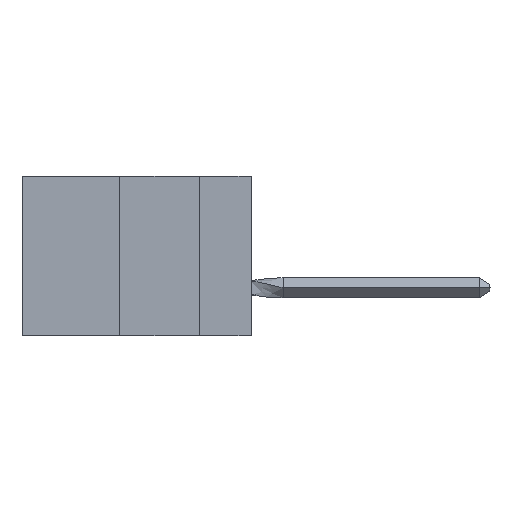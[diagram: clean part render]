
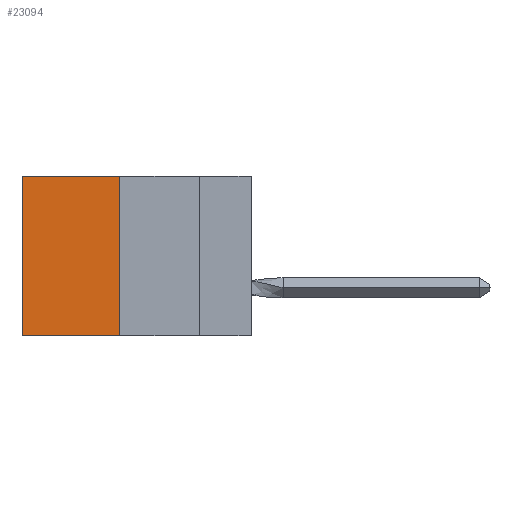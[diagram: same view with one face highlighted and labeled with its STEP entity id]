
A CAD part, left-side view. The second image highlights one B-rep face of the part: STEP entity #23094.
In plain terms, the highlighted planar face has unit normal (-1, 0, 0).
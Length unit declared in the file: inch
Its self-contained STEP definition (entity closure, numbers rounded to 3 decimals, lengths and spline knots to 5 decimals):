
#344 = CARTESIAN_POINT ( 'NONE',  ( 0.305, 0.413, -0.5 ) ) ;
#541 = CARTESIAN_POINT ( 'NONE',  ( 0.305, 0.72, 0. ) ) ;
#679 = DIRECTION ( 'NONE',  ( 0., 0., -1. ) ) ;
#1840 = DIRECTION ( 'NONE',  ( 0., 0., -1. ) ) ;
#2840 = VERTEX_POINT ( 'NONE', #541 ) ;
#3036 = CARTESIAN_POINT ( 'NONE',  ( 0.305, 0.413, 0. ) ) ;
#4230 = ORIENTED_EDGE ( 'NONE', *, *, #9345, .T. ) ;
#6288 = VERTEX_POINT ( 'NONE', #344 ) ;
#7302 = CARTESIAN_POINT ( 'NONE',  ( 0.305, 0.413, -0.5 ) ) ;
#7318 = CARTESIAN_POINT ( 'NONE',  ( 0.305, 0.413, -0.5 ) ) ;
#8744 = ORIENTED_EDGE ( 'NONE', *, *, #21693, .F. ) ;
#9033 = AXIS2_PLACEMENT_3D ( 'NONE', #7302, #18740, #679 ) ;
#9345 = EDGE_CURVE ( 'NONE', #17379, #2840, #23986, .T. ) ;
#9441 = CARTESIAN_POINT ( 'NONE',  ( 0.305, 0.72, -0.5 ) ) ;
#9584 = ORIENTED_EDGE ( 'NONE', *, *, #28906, .F. ) ;
#9917 = ORIENTED_EDGE ( 'NONE', *, *, #24493, .T. ) ;
#12864 = FACE_OUTER_BOUND ( 'NONE', #16783, .T. ) ;
#14125 = PLANE ( 'NONE',  #9033 ) ;
#16273 = DIRECTION ( 'NONE',  ( 0., 1., 0. ) ) ;
#16783 = EDGE_LOOP ( 'NONE', ( #9917, #9584, #8744, #4230 ) ) ;
#17379 = VERTEX_POINT ( 'NONE', #3036 ) ;
#18740 = DIRECTION ( 'NONE',  ( 1., 0., 0. ) ) ;
#18825 = CARTESIAN_POINT ( 'NONE',  ( 0.305, 0.72, -0.5 ) ) ;
#19716 = LINE ( 'NONE', #9441, #25693 ) ;
#20271 = CARTESIAN_POINT ( 'NONE',  ( 0.305, 0.413, 0. ) ) ;
#20462 = DIRECTION ( 'NONE',  ( 0., 1., 0. ) ) ;
#21693 = EDGE_CURVE ( 'NONE', #17379, #6288, #23740, .T. ) ;
#22146 = LINE ( 'NONE', #7318, #28485 ) ;
#22553 = VECTOR ( 'NONE', #20462, 39.37008 ) ;
#23094 = ADVANCED_FACE ( 'NONE', ( #12864 ), #14125, .F. ) ;
#23740 = LINE ( 'NONE', #24294, #26232 ) ;
#23986 = LINE ( 'NONE', #20271, #22553 ) ;
#24294 = CARTESIAN_POINT ( 'NONE',  ( 0.305, 0.413, -0.5 ) ) ;
#24493 = EDGE_CURVE ( 'NONE', #2840, #27118, #19716, .T. ) ;
#25057 = DIRECTION ( 'NONE',  ( 0., 0., -1. ) ) ;
#25693 = VECTOR ( 'NONE', #25057, 39.37008 ) ;
#26232 = VECTOR ( 'NONE', #1840, 39.37008 ) ;
#27118 = VERTEX_POINT ( 'NONE', #18825 ) ;
#28485 = VECTOR ( 'NONE', #16273, 39.37008 ) ;
#28906 = EDGE_CURVE ( 'NONE', #6288, #27118, #22146, .T. ) ;
